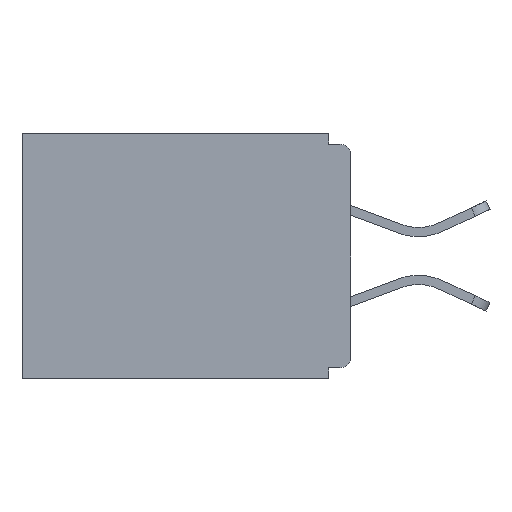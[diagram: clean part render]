
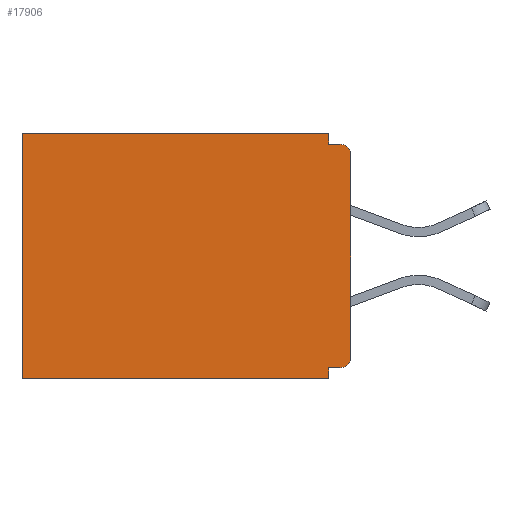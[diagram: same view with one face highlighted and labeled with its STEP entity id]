
A CAD part, left-side view. The second image highlights one B-rep face of the part: STEP entity #17906.
In plain terms, the highlighted planar face has unit normal (-1, 0, 0).
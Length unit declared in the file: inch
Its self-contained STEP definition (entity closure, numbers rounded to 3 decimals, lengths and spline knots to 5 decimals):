
#667 = CARTESIAN_POINT ( 'NONE',  ( 0.298, 0., -0.343 ) ) ;
#1019 = DIRECTION ( 'NONE',  ( 0., 0., -1. ) ) ;
#1245 = CARTESIAN_POINT ( 'NONE',  ( 0.298, 0.031, -0.343 ) ) ;
#1433 = ORIENTED_EDGE ( 'NONE', *, *, #4684, .F. ) ;
#1481 = CARTESIAN_POINT ( 'NONE',  ( 0.298, 0.015, -0.328 ) ) ;
#2112 = AXIS2_PLACEMENT_3D ( 'NONE', #4002, #12692, #13864 ) ;
#2122 = VERTEX_POINT ( 'NONE', #12129 ) ;
#2327 = ORIENTED_EDGE ( 'NONE', *, *, #16603, .T. ) ;
#2331 = CARTESIAN_POINT ( 'NONE',  ( 0.298, 0., -0.328 ) ) ;
#2839 = CARTESIAN_POINT ( 'NONE',  ( 0.298, 0.46, 0. ) ) ;
#3003 = CARTESIAN_POINT ( 'NONE',  ( 0.298, 0.015, -0.03 ) ) ;
#3056 = EDGE_CURVE ( 'NONE', #5166, #18162, #17838, .T. ) ;
#3446 = VECTOR ( 'NONE', #10435, 39.37008 ) ;
#3855 = CARTESIAN_POINT ( 'NONE',  ( 0.298, 0.46, 0. ) ) ;
#4002 = CARTESIAN_POINT ( 'NONE',  ( 0.298, 0.015, -0.313 ) ) ;
#4083 = EDGE_CURVE ( 'NONE', #13954, #11771, #9731, .T. ) ;
#4403 = CARTESIAN_POINT ( 'NONE',  ( 0.298, 0.031, -0.343 ) ) ;
#4552 = DIRECTION ( 'NONE',  ( 0., 0., -1. ) ) ;
#4684 = EDGE_CURVE ( 'NONE', #18162, #13195, #13746, .T. ) ;
#5029 = VERTEX_POINT ( 'NONE', #3855 ) ;
#5049 = VECTOR ( 'NONE', #5583, 39.37008 ) ;
#5158 = CARTESIAN_POINT ( 'NONE',  ( 0.298, 0., -0.03 ) ) ;
#5166 = VERTEX_POINT ( 'NONE', #1481 ) ;
#5187 = EDGE_LOOP ( 'NONE', ( #6341, #9411, #13181, #15600, #2327, #7103, #1433, #13588, #12932, #5537 ) ) ;
#5537 = ORIENTED_EDGE ( 'NONE', *, *, #4083, .F. ) ;
#5583 = DIRECTION ( 'NONE',  ( 0., -1., 0. ) ) ;
#5930 = CARTESIAN_POINT ( 'NONE',  ( 0.298, 0.015, -0.015 ) ) ;
#5961 = VECTOR ( 'NONE', #1019, 39.37008 ) ;
#6075 = DIRECTION ( 'NONE',  ( 0., 0., -1. ) ) ;
#6268 = CARTESIAN_POINT ( 'NONE',  ( 0.298, 0., 0. ) ) ;
#6341 = ORIENTED_EDGE ( 'NONE', *, *, #13301, .T. ) ;
#6985 = VECTOR ( 'NONE', #14226, 39.37008 ) ;
#7103 = ORIENTED_EDGE ( 'NONE', *, *, #11766, .F. ) ;
#7125 = VECTOR ( 'NONE', #6075, 39.37008 ) ;
#7157 = CIRCLE ( 'NONE', #2112, 0.015 ) ;
#7252 = PLANE ( 'NONE',  #12598 ) ;
#7268 = DIRECTION ( 'NONE',  ( -1., 0., 0. ) ) ;
#7619 = CARTESIAN_POINT ( 'NONE',  ( 0.298, 0., 0. ) ) ;
#9159 = EDGE_CURVE ( 'NONE', #5166, #11771, #7157, .T. ) ;
#9275 = LINE ( 'NONE', #15462, #5049 ) ;
#9411 = ORIENTED_EDGE ( 'NONE', *, *, #15345, .F. ) ;
#9731 = LINE ( 'NONE', #10490, #5961 ) ;
#10178 = EDGE_CURVE ( 'NONE', #2122, #11547, #16744, .T. ) ;
#10435 = DIRECTION ( 'NONE',  ( 0., 1., 0. ) ) ;
#10490 = CARTESIAN_POINT ( 'NONE',  ( 0.298, 0., 0. ) ) ;
#10502 = DIRECTION ( 'NONE',  ( 0., 0., -1. ) ) ;
#10534 = CARTESIAN_POINT ( 'NONE',  ( 0.298, 0., -0.313 ) ) ;
#10817 = VERTEX_POINT ( 'NONE', #5930 ) ;
#11328 = CARTESIAN_POINT ( 'NONE',  ( 0.298, 0.031, -0.328 ) ) ;
#11547 = VERTEX_POINT ( 'NONE', #14516 ) ;
#11698 = LINE ( 'NONE', #2839, #6985 ) ;
#11766 = EDGE_CURVE ( 'NONE', #13195, #14521, #14900, .T. ) ;
#11771 = VERTEX_POINT ( 'NONE', #10534 ) ;
#12129 = CARTESIAN_POINT ( 'NONE',  ( 0.298, 0.031, 0. ) ) ;
#12283 = DIRECTION ( 'NONE',  ( 0., 1., 0. ) ) ;
#12598 = AXIS2_PLACEMENT_3D ( 'NONE', #7619, #16337, #10502 ) ;
#12692 = DIRECTION ( 'NONE',  ( -1., 0., 0. ) ) ;
#12932 = ORIENTED_EDGE ( 'NONE', *, *, #9159, .T. ) ;
#13181 = ORIENTED_EDGE ( 'NONE', *, *, #10178, .F. ) ;
#13195 = VERTEX_POINT ( 'NONE', #16504 ) ;
#13224 = LINE ( 'NONE', #6268, #3446 ) ;
#13301 = EDGE_CURVE ( 'NONE', #13954, #10817, #14861, .T. ) ;
#13541 = VECTOR ( 'NONE', #12283, 39.37008 ) ;
#13588 = ORIENTED_EDGE ( 'NONE', *, *, #3056, .F. ) ;
#13746 = LINE ( 'NONE', #4403, #15736 ) ;
#13864 = DIRECTION ( 'NONE',  ( 0., 0., -1. ) ) ;
#13954 = VERTEX_POINT ( 'NONE', #5158 ) ;
#13961 = AXIS2_PLACEMENT_3D ( 'NONE', #3003, #7268, #4552 ) ;
#14202 = VECTOR ( 'NONE', #16323, 39.37008 ) ;
#14226 = DIRECTION ( 'NONE',  ( 0., 0., -1. ) ) ;
#14516 = CARTESIAN_POINT ( 'NONE',  ( 0.298, 0.031, -0.015 ) ) ;
#14521 = VERTEX_POINT ( 'NONE', #16601 ) ;
#14861 = CIRCLE ( 'NONE', #13961, 0.015 ) ;
#14900 = LINE ( 'NONE', #667, #13541 ) ;
#14994 = FACE_OUTER_BOUND ( 'NONE', #5187, .T. ) ;
#15345 = EDGE_CURVE ( 'NONE', #11547, #10817, #9275, .T. ) ;
#15462 = CARTESIAN_POINT ( 'NONE',  ( 0.298, 0., -0.015 ) ) ;
#15600 = ORIENTED_EDGE ( 'NONE', *, *, #17444, .T. ) ;
#15736 = VECTOR ( 'NONE', #17049, 39.37008 ) ;
#16323 = DIRECTION ( 'NONE',  ( 0., 1., 0. ) ) ;
#16337 = DIRECTION ( 'NONE',  ( 1., 0., 0. ) ) ;
#16504 = CARTESIAN_POINT ( 'NONE',  ( 0.298, 0.031, -0.343 ) ) ;
#16601 = CARTESIAN_POINT ( 'NONE',  ( 0.298, 0.46, -0.343 ) ) ;
#16603 = EDGE_CURVE ( 'NONE', #5029, #14521, #11698, .T. ) ;
#16744 = LINE ( 'NONE', #1245, #7125 ) ;
#17049 = DIRECTION ( 'NONE',  ( 0., 0., -1. ) ) ;
#17444 = EDGE_CURVE ( 'NONE', #2122, #5029, #13224, .T. ) ;
#17838 = LINE ( 'NONE', #2331, #14202 ) ;
#17906 = ADVANCED_FACE ( 'NONE', ( #14994 ), #7252, .F. ) ;
#18162 = VERTEX_POINT ( 'NONE', #11328 ) ;
